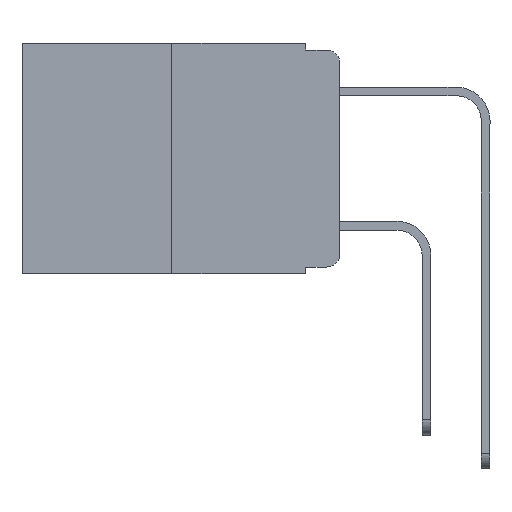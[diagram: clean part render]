
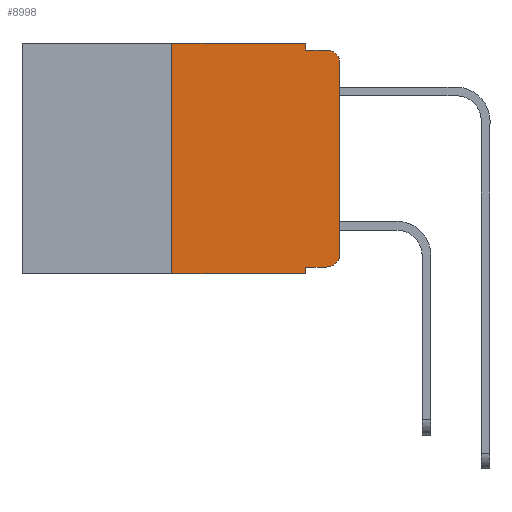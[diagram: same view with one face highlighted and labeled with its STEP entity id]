
A CAD part, left-side view. The second image highlights one B-rep face of the part: STEP entity #8998.
In plain terms, the highlighted planar face has unit normal (-1, 0, 0).
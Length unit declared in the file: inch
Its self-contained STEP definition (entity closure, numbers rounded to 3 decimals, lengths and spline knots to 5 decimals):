
#74 = DIRECTION ( 'NONE',  ( 0., -1., 0. ) ) ;
#132 = VERTEX_POINT ( 'NONE', #6731 ) ;
#287 = FACE_OUTER_BOUND ( 'NONE', #3661, .T. ) ;
#352 = CARTESIAN_POINT ( 'NONE',  ( 0., 0.051, -0.333 ) ) ;
#465 = DIRECTION ( 'NONE',  ( 0., 0., -1. ) ) ;
#500 = DIRECTION ( 'NONE',  ( 0., -1., 0. ) ) ;
#638 = ORIENTED_EDGE ( 'NONE', *, *, #7917, .T. ) ;
#939 = DIRECTION ( 'NONE',  ( 0., 0., 1. ) ) ;
#1216 = LINE ( 'NONE', #5235, #9440 ) ;
#1427 = CIRCLE ( 'NONE', #3955, 0.02 ) ;
#1435 = AXIS2_PLACEMENT_3D ( 'NONE', #2191, #10113, #3381 ) ;
#1616 = CIRCLE ( 'NONE', #1435, 0.02 ) ;
#2012 = CARTESIAN_POINT ( 'NONE',  ( 0., 0.051, -0.333 ) ) ;
#2191 = CARTESIAN_POINT ( 'NONE',  ( 0., 0.02, -0.03 ) ) ;
#2741 = DIRECTION ( 'NONE',  ( 0., -1., 0. ) ) ;
#2804 = VERTEX_POINT ( 'NONE', #13963 ) ;
#2936 = LINE ( 'NONE', #9139, #11474 ) ;
#2981 = EDGE_CURVE ( 'NONE', #13218, #8426, #1427, .T. ) ;
#3254 = EDGE_CURVE ( 'NONE', #3662, #3701, #1216, .T. ) ;
#3381 = DIRECTION ( 'NONE',  ( 0., 0., -1. ) ) ;
#3661 = EDGE_LOOP ( 'NONE', ( #5638, #11749, #14482, #6350, #6711, #9653, #638, #9953, #12714, #10282 ) ) ;
#3662 = VERTEX_POINT ( 'NONE', #13876 ) ;
#3701 = VERTEX_POINT ( 'NONE', #7716 ) ;
#3955 = AXIS2_PLACEMENT_3D ( 'NONE', #12674, #10114, #10207 ) ;
#4334 = CARTESIAN_POINT ( 'NONE',  ( 0., 0.051, -0.343 ) ) ;
#4402 = CARTESIAN_POINT ( 'NONE',  ( 0., 0., 0. ) ) ;
#4437 = VECTOR ( 'NONE', #9005, 39.37008 ) ;
#4789 = EDGE_CURVE ( 'NONE', #3701, #7726, #13094, .T. ) ;
#4843 = CARTESIAN_POINT ( 'NONE',  ( 0., 0., -0.03 ) ) ;
#4870 = CARTESIAN_POINT ( 'NONE',  ( 0., 0.051, -0.01 ) ) ;
#5235 = CARTESIAN_POINT ( 'NONE',  ( 0., 0.473, 0. ) ) ;
#5343 = EDGE_CURVE ( 'NONE', #12510, #13218, #9240, .T. ) ;
#5380 = VECTOR ( 'NONE', #500, 39.37008 ) ;
#5546 = EDGE_CURVE ( 'NONE', #132, #3662, #2936, .T. ) ;
#5638 = ORIENTED_EDGE ( 'NONE', *, *, #11981, .T. ) ;
#6007 = VECTOR ( 'NONE', #7167, 39.37008 ) ;
#6350 = ORIENTED_EDGE ( 'NONE', *, *, #4789, .F. ) ;
#6601 = VERTEX_POINT ( 'NONE', #4334 ) ;
#6711 = ORIENTED_EDGE ( 'NONE', *, *, #3254, .F. ) ;
#6716 = DIRECTION ( 'NONE',  ( 0., 0., 1. ) ) ;
#6731 = CARTESIAN_POINT ( 'NONE',  ( 0., 0.25, -0.343 ) ) ;
#6844 = DIRECTION ( 'NONE',  ( 0., 0., -1. ) ) ;
#7167 = DIRECTION ( 'NONE',  ( 0., -1., 0. ) ) ;
#7273 = CARTESIAN_POINT ( 'NONE',  ( 0., 0.051, -0.01 ) ) ;
#7626 = VERTEX_POINT ( 'NONE', #4843 ) ;
#7670 = DIRECTION ( 'NONE',  ( 1., 0., 0. ) ) ;
#7716 = CARTESIAN_POINT ( 'NONE',  ( 0., 0.051, 0. ) ) ;
#7726 = VERTEX_POINT ( 'NONE', #7273 ) ;
#7917 = EDGE_CURVE ( 'NONE', #132, #6601, #11187, .T. ) ;
#8046 = AXIS2_PLACEMENT_3D ( 'NONE', #13962, #7670, #465 ) ;
#8426 = VERTEX_POINT ( 'NONE', #13978 ) ;
#8640 = CARTESIAN_POINT ( 'NONE',  ( 0., 0.02, -0.333 ) ) ;
#8998 = ADVANCED_FACE ( 'NONE', ( #287 ), #9807, .F. ) ;
#9005 = DIRECTION ( 'NONE',  ( 0., 0., -1. ) ) ;
#9127 = EDGE_CURVE ( 'NONE', #7626, #2804, #1616, .T. ) ;
#9139 = CARTESIAN_POINT ( 'NONE',  ( 0., 0.25, 0. ) ) ;
#9143 = EDGE_CURVE ( 'NONE', #12510, #6601, #10359, .T. ) ;
#9240 = LINE ( 'NONE', #2012, #10984 ) ;
#9440 = VECTOR ( 'NONE', #74, 39.37008 ) ;
#9508 = LINE ( 'NONE', #4402, #11925 ) ;
#9653 = ORIENTED_EDGE ( 'NONE', *, *, #5546, .F. ) ;
#9807 = PLANE ( 'NONE',  #8046 ) ;
#9953 = ORIENTED_EDGE ( 'NONE', *, *, #9143, .F. ) ;
#10113 = DIRECTION ( 'NONE',  ( -1., 0., 0. ) ) ;
#10114 = DIRECTION ( 'NONE',  ( -1., 0., 0. ) ) ;
#10207 = DIRECTION ( 'NONE',  ( 0., 0., -1. ) ) ;
#10282 = ORIENTED_EDGE ( 'NONE', *, *, #2981, .T. ) ;
#10359 = LINE ( 'NONE', #12208, #13112 ) ;
#10523 = CARTESIAN_POINT ( 'NONE',  ( 0., 0.051, 0. ) ) ;
#10984 = VECTOR ( 'NONE', #2741, 39.37008 ) ;
#11187 = LINE ( 'NONE', #12950, #5380 ) ;
#11474 = VECTOR ( 'NONE', #939, 39.37008 ) ;
#11749 = ORIENTED_EDGE ( 'NONE', *, *, #9127, .T. ) ;
#11925 = VECTOR ( 'NONE', #6716, 39.37008 ) ;
#11981 = EDGE_CURVE ( 'NONE', #8426, #7626, #9508, .T. ) ;
#12208 = CARTESIAN_POINT ( 'NONE',  ( 0., 0.051, 0. ) ) ;
#12237 = EDGE_CURVE ( 'NONE', #7726, #2804, #14488, .T. ) ;
#12510 = VERTEX_POINT ( 'NONE', #352 ) ;
#12674 = CARTESIAN_POINT ( 'NONE',  ( 0., 0.02, -0.313 ) ) ;
#12714 = ORIENTED_EDGE ( 'NONE', *, *, #5343, .T. ) ;
#12950 = CARTESIAN_POINT ( 'NONE',  ( 0., 0.473, -0.343 ) ) ;
#13094 = LINE ( 'NONE', #10523, #4437 ) ;
#13112 = VECTOR ( 'NONE', #6844, 39.37008 ) ;
#13218 = VERTEX_POINT ( 'NONE', #8640 ) ;
#13876 = CARTESIAN_POINT ( 'NONE',  ( 0., 0.25, 0. ) ) ;
#13962 = CARTESIAN_POINT ( 'NONE',  ( 0., 0.473, 0. ) ) ;
#13963 = CARTESIAN_POINT ( 'NONE',  ( 0., 0.02, -0.01 ) ) ;
#13978 = CARTESIAN_POINT ( 'NONE',  ( 0., 0., -0.313 ) ) ;
#14482 = ORIENTED_EDGE ( 'NONE', *, *, #12237, .F. ) ;
#14488 = LINE ( 'NONE', #4870, #6007 ) ;
